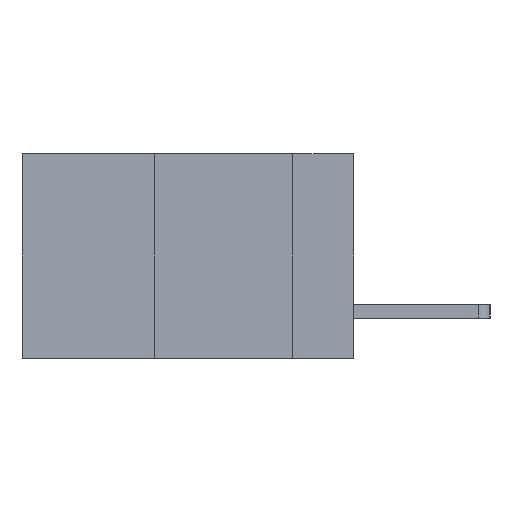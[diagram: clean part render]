
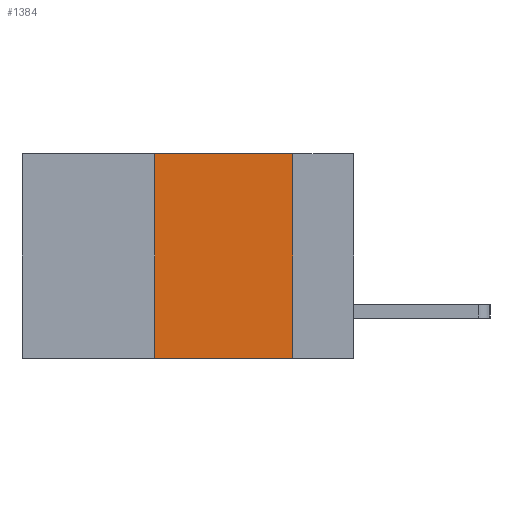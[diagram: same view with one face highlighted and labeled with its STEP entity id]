
A CAD part, left-side view. The second image highlights one B-rep face of the part: STEP entity #1384.
In plain terms, the highlighted planar face has unit normal (-1, 0, 0).
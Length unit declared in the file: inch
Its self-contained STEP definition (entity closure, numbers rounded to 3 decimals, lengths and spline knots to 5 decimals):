
#359 = EDGE_CURVE ( 'NONE', #9175, #3025, #10930, .T. ) ;
#823 = VECTOR ( 'NONE', #10105, 39.37008 ) ;
#1197 = CARTESIAN_POINT ( 'NONE',  ( 0., 0.6, 0. ) ) ;
#1334 = EDGE_LOOP ( 'NONE', ( #5640, #6890, #7292, #9434 ) ) ;
#1384 = ADVANCED_FACE ( 'NONE', ( #8374 ), #3804, .F. ) ;
#1726 = DIRECTION ( 'NONE',  ( 1., 0., 0. ) ) ;
#2424 = DIRECTION ( 'NONE',  ( 0., 0., 1. ) ) ;
#2752 = VECTOR ( 'NONE', #9105, 39.37008 ) ;
#3025 = VERTEX_POINT ( 'NONE', #4740 ) ;
#3804 = PLANE ( 'NONE',  #4833 ) ;
#4512 = CARTESIAN_POINT ( 'NONE',  ( 0., 0.6, 0. ) ) ;
#4723 = CARTESIAN_POINT ( 'NONE',  ( 0., 0.36, -0.37 ) ) ;
#4740 = CARTESIAN_POINT ( 'NONE',  ( 0., 0.11, -0.37 ) ) ;
#4833 = AXIS2_PLACEMENT_3D ( 'NONE', #4512, #1726, #6528 ) ;
#5640 = ORIENTED_EDGE ( 'NONE', *, *, #359, .F. ) ;
#5673 = CARTESIAN_POINT ( 'NONE',  ( 0., 0.6, -0.37 ) ) ;
#5703 = CARTESIAN_POINT ( 'NONE',  ( 0., 0.36, 0. ) ) ;
#5858 = CARTESIAN_POINT ( 'NONE',  ( 0., 0.11, 0. ) ) ;
#5918 = VECTOR ( 'NONE', #7438, 39.37008 ) ;
#6024 = EDGE_CURVE ( 'NONE', #11792, #11200, #12080, .T. ) ;
#6132 = CARTESIAN_POINT ( 'NONE',  ( 0., 0.11, 0. ) ) ;
#6243 = LINE ( 'NONE', #1197, #823 ) ;
#6528 = DIRECTION ( 'NONE',  ( 0., 0., -1. ) ) ;
#6890 = ORIENTED_EDGE ( 'NONE', *, *, #11562, .F. ) ;
#7271 = CARTESIAN_POINT ( 'NONE',  ( 0., 0.36, 0. ) ) ;
#7292 = ORIENTED_EDGE ( 'NONE', *, *, #6024, .F. ) ;
#7438 = DIRECTION ( 'NONE',  ( 0., -1., 0. ) ) ;
#8374 = FACE_OUTER_BOUND ( 'NONE', #1334, .T. ) ;
#8522 = LINE ( 'NONE', #5673, #5918 ) ;
#9033 = EDGE_CURVE ( 'NONE', #11792, #3025, #8522, .T. ) ;
#9105 = DIRECTION ( 'NONE',  ( 0., 0., -1. ) ) ;
#9175 = VERTEX_POINT ( 'NONE', #5858 ) ;
#9401 = VECTOR ( 'NONE', #2424, 39.37008 ) ;
#9434 = ORIENTED_EDGE ( 'NONE', *, *, #9033, .T. ) ;
#10105 = DIRECTION ( 'NONE',  ( 0., -1., 0. ) ) ;
#10930 = LINE ( 'NONE', #6132, #2752 ) ;
#11200 = VERTEX_POINT ( 'NONE', #5703 ) ;
#11562 = EDGE_CURVE ( 'NONE', #11200, #9175, #6243, .T. ) ;
#11792 = VERTEX_POINT ( 'NONE', #4723 ) ;
#12080 = LINE ( 'NONE', #7271, #9401 ) ;
